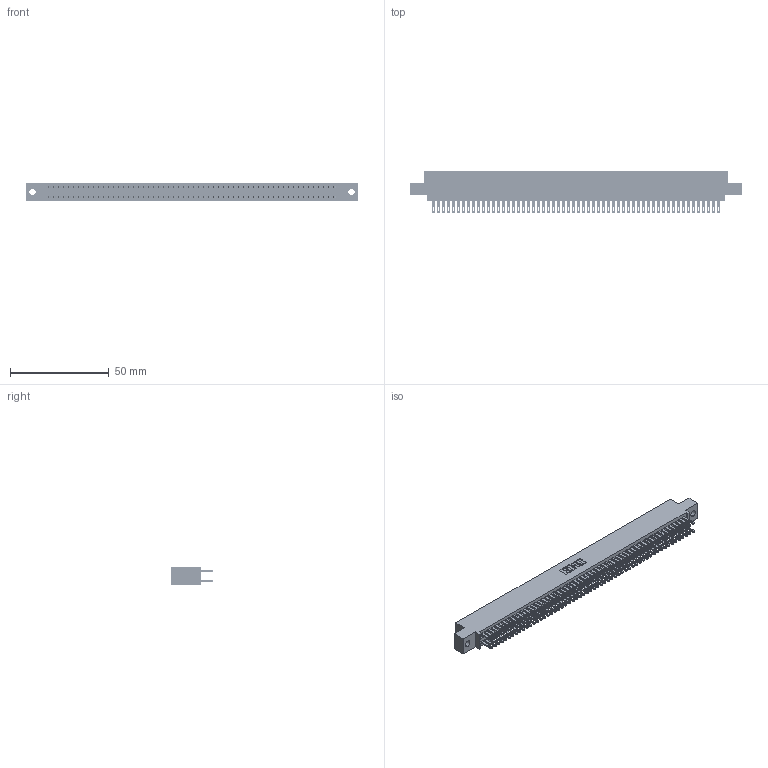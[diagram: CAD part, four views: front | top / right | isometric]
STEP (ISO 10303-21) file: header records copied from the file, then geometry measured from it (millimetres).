
FILE_DESCRIPTION (( 'STEP AP203' ), '1' );
FILE_NAME ('345-116-500-502.STEP', '2019-11-05T13:35:59', ( '' ), ( '' ), 'SwSTEP 2.0', 'SolidWorks 2016', '' );
FILE_SCHEMA (( 'CONFIG_CONTROL_DESIGN' ));
Length unit declared in the file: inch
Products named in the file (3): 345-292-001_345-293-100; 345 Part_0.110 Offset - 0.128 Dia; 345-116-500-502
Assembly tree (117 placements, depth 2):
  345-116-500-502
    345 Part_0.110 Offset - 0.128 Dia
    345-292-001_345-293-100  x116
Bounding box: 168.53 x 21.51 x 9.4 mm (x, y, z)
Volume: 16764 mm3; surface area: 26093.2 mm2
Topology: 117 solids, 117 shells, 5466 faces, 16709 edges, 11138 vertices
Faces by surface type: plane 3216, cylinder 2250
Entity records: 43419 total; most frequent: CARTESIAN_POINT 7264, ORIENTED_EDGE 7198, DIRECTION 6387, EDGE_CURVE 3599, VECTOR 3231, LINE 3231, VERTEX_POINT 2398, AXIS2_PLACEMENT_3D 1578
